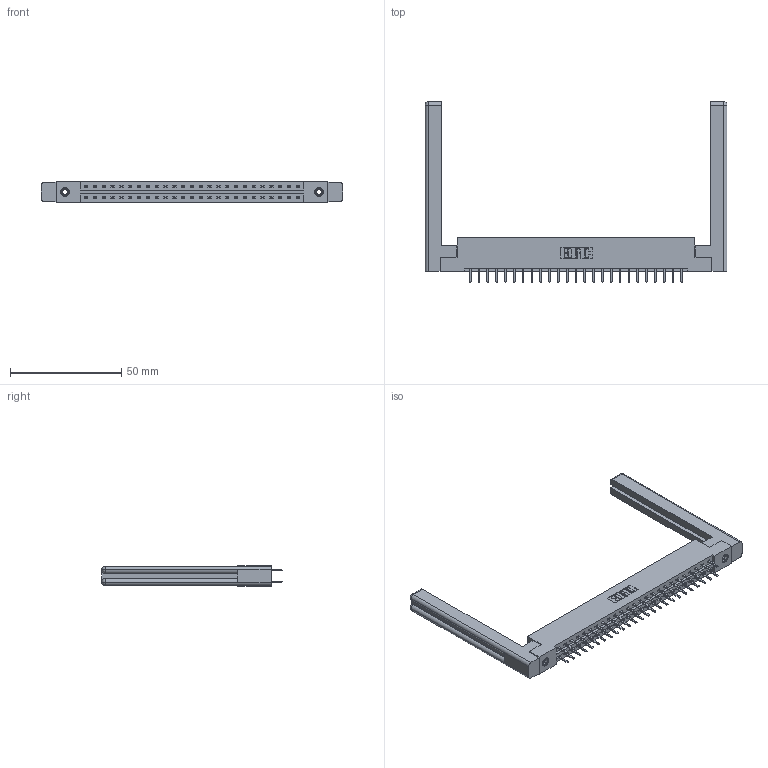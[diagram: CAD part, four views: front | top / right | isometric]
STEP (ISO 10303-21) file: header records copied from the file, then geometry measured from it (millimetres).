
FILE_DESCRIPTION (( 'STEP AP203' ), '1' );
FILE_NAME ('337-050-520-258.STEP', '2019-10-09T15:31:00', ( '' ), ( '' ), 'SwSTEP 2.0', 'SolidWorks 2016', '' );
FILE_SCHEMA (( 'CONFIG_CONTROL_DESIGN' ));
Length unit declared in the file: inch
Products named in the file (5): 337 Part_Flush Mounting Lugs - 0.156 Dia-TI; 345-250-001_345-250-001-102; 337-050-520-258; 345-292-001_345-293-120; 307-220-058
Assembly tree (55 placements, depth 2):
  337-050-520-258
    337 Part_Flush Mounting Lugs - 0.156 Dia-TI
    345-292-001_345-293-120  x50
    345-250-001_345-250-001-102  x2
    307-220-058  x2
Bounding box: 135.69 x 81.11 x 9.4 mm (x, y, z)
Volume: 21193.8 mm3; surface area: 20704.2 mm2
Topology: 55 solids, 55 shells, 3156 faces, 9115 edges, 5930 vertices
Faces by surface type: plane 2154, cylinder 978, cone 12, torus 12
Entity records: 24330 total; most frequent: CARTESIAN_POINT 4133, ORIENTED_EDGE 3996, DIRECTION 3550, EDGE_CURVE 1998, LINE 1818, VECTOR 1818, VERTEX_POINT 1322, AXIS2_PLACEMENT_3D 866
